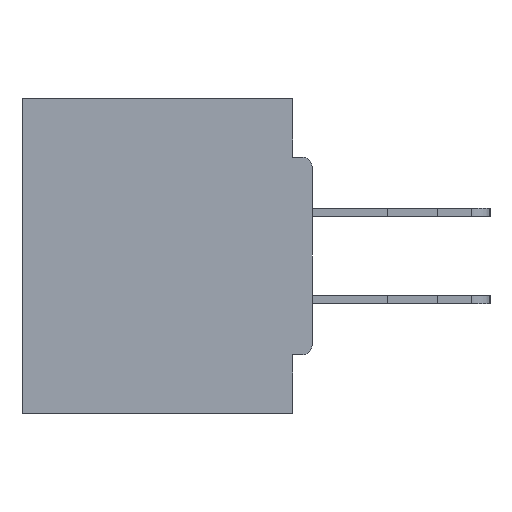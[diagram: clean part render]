
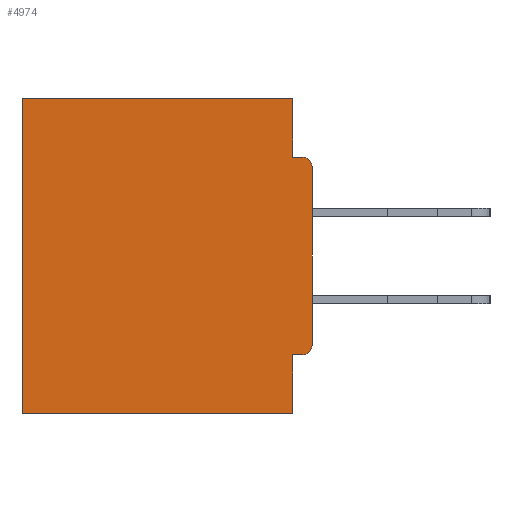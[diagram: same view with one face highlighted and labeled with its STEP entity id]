
A CAD part, left-side view. The second image highlights one B-rep face of the part: STEP entity #4974.
In plain terms, the highlighted planar face has unit normal (-1, 0, 0).
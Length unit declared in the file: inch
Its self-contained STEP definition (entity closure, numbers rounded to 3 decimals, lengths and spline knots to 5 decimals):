
#238 = CARTESIAN_POINT ( 'NONE',  ( 0.298, 0., -0.1085 ) ) ;
#496 = FACE_OUTER_BOUND ( 'NONE', #9445, .T. ) ;
#595 = EDGE_CURVE ( 'NONE', #16442, #18800, #30079, .T. ) ;
#654 = EDGE_CURVE ( 'NONE', #787, #8235, #38244, .T. ) ;
#787 = VERTEX_POINT ( 'NONE', #13340 ) ;
#993 = AXIS2_PLACEMENT_3D ( 'NONE', #25271, #25003, #12946 ) ;
#1910 = EDGE_CURVE ( 'NONE', #20207, #18800, #8702, .T. ) ;
#2043 = CARTESIAN_POINT ( 'NONE',  ( 0.298, 0., -0.3915 ) ) ;
#2272 = DIRECTION ( 'NONE',  ( 0., 0., -1. ) ) ;
#3568 = DIRECTION ( 'NONE',  ( -1., 0., 0. ) ) ;
#4322 = DIRECTION ( 'NONE',  ( 0., 1., 0. ) ) ;
#4974 = ADVANCED_FACE ( 'NONE', ( #496 ), #38348, .F. ) ;
#5812 = LINE ( 'NONE', #27790, #33459 ) ;
#6113 = ORIENTED_EDGE ( 'NONE', *, *, #654, .F. ) ;
#7604 = ORIENTED_EDGE ( 'NONE', *, *, #24282, .F. ) ;
#8170 = VECTOR ( 'NONE', #2272, 39.37008 ) ;
#8235 = VERTEX_POINT ( 'NONE', #8692 ) ;
#8326 = EDGE_CURVE ( 'NONE', #16442, #8235, #14590, .T. ) ;
#8692 = CARTESIAN_POINT ( 'NONE',  ( 0.298, 0.015, -0.0935 ) ) ;
#8702 = CIRCLE ( 'NONE', #993, 0.015 ) ;
#9207 = DIRECTION ( 'NONE',  ( 0., 1., 0. ) ) ;
#9445 = EDGE_LOOP ( 'NONE', ( #34946, #6113, #37681, #16314, #19462, #24904, #38552, #7604, #33177, #35499 ) ) ;
#9632 = CARTESIAN_POINT ( 'NONE',  ( 0.298, 0.015, -0.1085 ) ) ;
#10554 = LINE ( 'NONE', #17062, #17099 ) ;
#10951 = VERTEX_POINT ( 'NONE', #14211 ) ;
#12274 = DIRECTION ( 'NONE',  ( 0., 0., -1. ) ) ;
#12569 = VECTOR ( 'NONE', #14328, 39.37008 ) ;
#12946 = DIRECTION ( 'NONE',  ( 0., 0., -1. ) ) ;
#13207 = CARTESIAN_POINT ( 'NONE',  ( 0.298, 0.46, -0.5 ) ) ;
#13311 = CARTESIAN_POINT ( 'NONE',  ( 0.298, 0.031, -0.5 ) ) ;
#13340 = CARTESIAN_POINT ( 'NONE',  ( 0.298, 0.031, -0.0935 ) ) ;
#13565 = CARTESIAN_POINT ( 'NONE',  ( 0.298, 0., -0.4065 ) ) ;
#13616 = EDGE_CURVE ( 'NONE', #10951, #787, #16231, .T. ) ;
#14211 = CARTESIAN_POINT ( 'NONE',  ( 0.298, 0.031, 0. ) ) ;
#14328 = DIRECTION ( 'NONE',  ( 0., 1., 0. ) ) ;
#14465 = DIRECTION ( 'NONE',  ( 1., 0., 0. ) ) ;
#14590 = CIRCLE ( 'NONE', #27545, 0.015 ) ;
#16231 = LINE ( 'NONE', #20573, #8170 ) ;
#16314 = ORIENTED_EDGE ( 'NONE', *, *, #36420, .T. ) ;
#16442 = VERTEX_POINT ( 'NONE', #238 ) ;
#16655 = CARTESIAN_POINT ( 'NONE',  ( 0.298, 0.46, 0. ) ) ;
#17062 = CARTESIAN_POINT ( 'NONE',  ( 0.298, 0.031, -0.5 ) ) ;
#17099 = VECTOR ( 'NONE', #32029, 39.37008 ) ;
#17594 = VERTEX_POINT ( 'NONE', #13311 ) ;
#17935 = EDGE_CURVE ( 'NONE', #38026, #37429, #21118, .T. ) ;
#18486 = CARTESIAN_POINT ( 'NONE',  ( 0.298, 0.46, 0. ) ) ;
#18671 = CARTESIAN_POINT ( 'NONE',  ( 0.298, 0.031, -0.4065 ) ) ;
#18800 = VERTEX_POINT ( 'NONE', #2043 ) ;
#19335 = DIRECTION ( 'NONE',  ( 0., 0., -1. ) ) ;
#19462 = ORIENTED_EDGE ( 'NONE', *, *, #17935, .T. ) ;
#20207 = VERTEX_POINT ( 'NONE', #27409 ) ;
#20573 = CARTESIAN_POINT ( 'NONE',  ( 0.298, 0.031, -0.5 ) ) ;
#21118 = LINE ( 'NONE', #16655, #29242 ) ;
#22007 = VERTEX_POINT ( 'NONE', #18671 ) ;
#23856 = CARTESIAN_POINT ( 'NONE',  ( 0.298, 0., -0.5 ) ) ;
#24047 = AXIS2_PLACEMENT_3D ( 'NONE', #29613, #14465, #35772 ) ;
#24084 = CARTESIAN_POINT ( 'NONE',  ( 0.298, 0., 0. ) ) ;
#24282 = EDGE_CURVE ( 'NONE', #20207, #22007, #24495, .T. ) ;
#24418 = LINE ( 'NONE', #23856, #12569 ) ;
#24495 = LINE ( 'NONE', #13565, #26412 ) ;
#24627 = DIRECTION ( 'NONE',  ( 0., 0., -1. ) ) ;
#24904 = ORIENTED_EDGE ( 'NONE', *, *, #25118, .F. ) ;
#25003 = DIRECTION ( 'NONE',  ( -1., 0., 0. ) ) ;
#25118 = EDGE_CURVE ( 'NONE', #17594, #37429, #24418, .T. ) ;
#25271 = CARTESIAN_POINT ( 'NONE',  ( 0.298, 0.015, -0.3915 ) ) ;
#26412 = VECTOR ( 'NONE', #4322, 39.37008 ) ;
#27409 = CARTESIAN_POINT ( 'NONE',  ( 0.298, 0.015, -0.4065 ) ) ;
#27545 = AXIS2_PLACEMENT_3D ( 'NONE', #9632, #3568, #12274 ) ;
#27573 = DIRECTION ( 'NONE',  ( 0., -1., 0. ) ) ;
#27790 = CARTESIAN_POINT ( 'NONE',  ( 0.298, 0., 0. ) ) ;
#29242 = VECTOR ( 'NONE', #19335, 39.37008 ) ;
#29613 = CARTESIAN_POINT ( 'NONE',  ( 0.298, 0., 0. ) ) ;
#30079 = LINE ( 'NONE', #24084, #36308 ) ;
#31915 = EDGE_CURVE ( 'NONE', #22007, #17594, #10554, .T. ) ;
#32029 = DIRECTION ( 'NONE',  ( 0., 0., -1. ) ) ;
#33177 = ORIENTED_EDGE ( 'NONE', *, *, #1910, .T. ) ;
#33459 = VECTOR ( 'NONE', #9207, 39.37008 ) ;
#34946 = ORIENTED_EDGE ( 'NONE', *, *, #8326, .T. ) ;
#35499 = ORIENTED_EDGE ( 'NONE', *, *, #595, .F. ) ;
#35772 = DIRECTION ( 'NONE',  ( 0., 0., -1. ) ) ;
#36308 = VECTOR ( 'NONE', #24627, 39.37008 ) ;
#36420 = EDGE_CURVE ( 'NONE', #10951, #38026, #5812, .T. ) ;
#36556 = CARTESIAN_POINT ( 'NONE',  ( 0.298, 0., -0.0935 ) ) ;
#37429 = VERTEX_POINT ( 'NONE', #13207 ) ;
#37681 = ORIENTED_EDGE ( 'NONE', *, *, #13616, .F. ) ;
#38026 = VERTEX_POINT ( 'NONE', #18486 ) ;
#38244 = LINE ( 'NONE', #36556, #38718 ) ;
#38348 = PLANE ( 'NONE',  #24047 ) ;
#38552 = ORIENTED_EDGE ( 'NONE', *, *, #31915, .F. ) ;
#38718 = VECTOR ( 'NONE', #27573, 39.37008 ) ;
